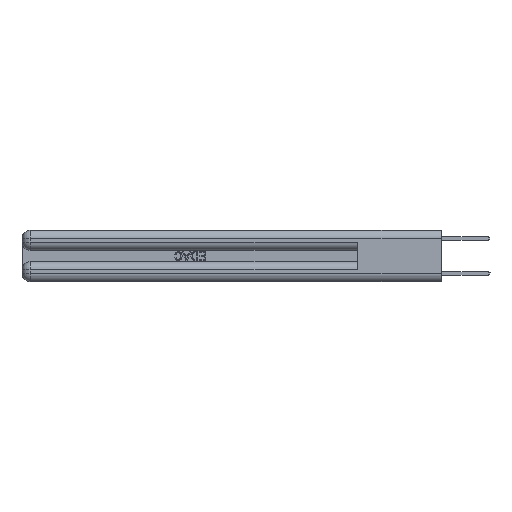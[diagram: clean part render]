
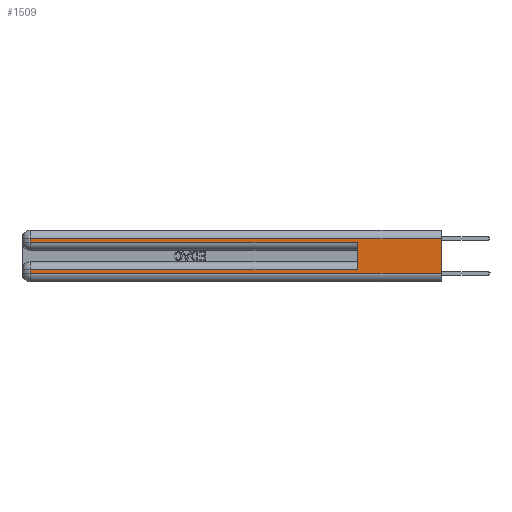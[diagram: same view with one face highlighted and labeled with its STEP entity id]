
A CAD part, left-side view. The second image highlights one B-rep face of the part: STEP entity #1509.
In plain terms, the highlighted planar face has unit normal (-1, 0, 0).
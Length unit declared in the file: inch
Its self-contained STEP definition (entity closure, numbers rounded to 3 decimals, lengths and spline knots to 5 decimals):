
#1509 = ADVANCED_FACE ( 'NONE', ( #26019 ), #21164, .F. ) ;
#1555 = VECTOR ( 'NONE', #27478, 39.37008 ) ;
#2676 = ORIENTED_EDGE ( 'NONE', *, *, #32297, .T. ) ;
#3340 = LINE ( 'NONE', #23990, #4583 ) ;
#3358 = VERTEX_POINT ( 'NONE', #25295 ) ;
#4510 = VECTOR ( 'NONE', #8321, 39.37008 ) ;
#4583 = VECTOR ( 'NONE', #26421, 39.37008 ) ;
#4674 = LINE ( 'NONE', #17213, #26048 ) ;
#5119 = VERTEX_POINT ( 'NONE', #22044 ) ;
#5182 = CARTESIAN_POINT ( 'NONE',  ( 0., 0., 0.31 ) ) ;
#6257 = DIRECTION ( 'NONE',  ( 0., 0., 1. ) ) ;
#6576 = ORIENTED_EDGE ( 'NONE', *, *, #20934, .T. ) ;
#8011 = AXIS2_PLACEMENT_3D ( 'NONE', #23850, #18541, #18206 ) ;
#8321 = DIRECTION ( 'NONE',  ( 0., 1., 0. ) ) ;
#9750 = CARTESIAN_POINT ( 'NONE',  ( 0., 2.94, 0.285 ) ) ;
#9998 = CARTESIAN_POINT ( 'NONE',  ( 0., 2.94, 0.06 ) ) ;
#10073 = LINE ( 'NONE', #34073, #13478 ) ;
#10141 = ORIENTED_EDGE ( 'NONE', *, *, #14459, .T. ) ;
#10171 = VERTEX_POINT ( 'NONE', #15647 ) ;
#10617 = VERTEX_POINT ( 'NONE', #9750 ) ;
#11072 = CARTESIAN_POINT ( 'NONE',  ( 0., 0., 0.285 ) ) ;
#11188 = DIRECTION ( 'NONE',  ( 0., -1., 0. ) ) ;
#11215 = ORIENTED_EDGE ( 'NONE', *, *, #25779, .T. ) ;
#11703 = CARTESIAN_POINT ( 'NONE',  ( 0., 0.6, 0.285 ) ) ;
#12539 = CARTESIAN_POINT ( 'NONE',  ( 0., 0.6, 0.085 ) ) ;
#13371 = ORIENTED_EDGE ( 'NONE', *, *, #18520, .F. ) ;
#13478 = VECTOR ( 'NONE', #25887, 39.37008 ) ;
#13658 = ORIENTED_EDGE ( 'NONE', *, *, #30019, .F. ) ;
#13848 = VECTOR ( 'NONE', #18808, 39.37008 ) ;
#13983 = VECTOR ( 'NONE', #29239, 39.37008 ) ;
#14459 = EDGE_CURVE ( 'NONE', #27688, #10171, #24209, .T. ) ;
#15647 = CARTESIAN_POINT ( 'NONE',  ( 0., 2.94, 0.085 ) ) ;
#15725 = EDGE_LOOP ( 'NONE', ( #13658, #6576, #2676, #28326, #13371, #10141, #11215, #18816 ) ) ;
#16240 = CARTESIAN_POINT ( 'NONE',  ( 0., 0., 0.085 ) ) ;
#16545 = LINE ( 'NONE', #18917, #13983 ) ;
#17213 = CARTESIAN_POINT ( 'NONE',  ( 0., 0.6, 0.145 ) ) ;
#18206 = DIRECTION ( 'NONE',  ( 0., 0., -1. ) ) ;
#18520 = EDGE_CURVE ( 'NONE', #27688, #21229, #4674, .T. ) ;
#18541 = DIRECTION ( 'NONE',  ( 1., 0., 0. ) ) ;
#18808 = DIRECTION ( 'NONE',  ( 0., 0., -1. ) ) ;
#18816 = ORIENTED_EDGE ( 'NONE', *, *, #27837, .T. ) ;
#18917 = CARTESIAN_POINT ( 'NONE',  ( 0., 0., 0.37 ) ) ;
#20900 = LINE ( 'NONE', #30512, #1555 ) ;
#20934 = EDGE_CURVE ( 'NONE', #26578, #3358, #3340, .T. ) ;
#21164 = PLANE ( 'NONE',  #8011 ) ;
#21229 = VERTEX_POINT ( 'NONE', #11703 ) ;
#22044 = CARTESIAN_POINT ( 'NONE',  ( 0., 0., 0.06 ) ) ;
#22834 = LINE ( 'NONE', #11072, #26942 ) ;
#23850 = CARTESIAN_POINT ( 'NONE',  ( 0., 0., 0.37 ) ) ;
#23990 = CARTESIAN_POINT ( 'NONE',  ( 0., 0., 0.31 ) ) ;
#24209 = LINE ( 'NONE', #16240, #4510 ) ;
#25295 = CARTESIAN_POINT ( 'NONE',  ( 0., 2.94, 0.31 ) ) ;
#25779 = EDGE_CURVE ( 'NONE', #10171, #33607, #10073, .T. ) ;
#25887 = DIRECTION ( 'NONE',  ( 0., 0., -1. ) ) ;
#26019 = FACE_OUTER_BOUND ( 'NONE', #15725, .T. ) ;
#26048 = VECTOR ( 'NONE', #6257, 39.37008 ) ;
#26421 = DIRECTION ( 'NONE',  ( 0., 1., 0. ) ) ;
#26578 = VERTEX_POINT ( 'NONE', #5182 ) ;
#26768 = CARTESIAN_POINT ( 'NONE',  ( 0., 2.94, 0.37 ) ) ;
#26942 = VECTOR ( 'NONE', #11188, 39.37008 ) ;
#27478 = DIRECTION ( 'NONE',  ( 0., -1., 0. ) ) ;
#27688 = VERTEX_POINT ( 'NONE', #12539 ) ;
#27837 = EDGE_CURVE ( 'NONE', #33607, #5119, #20900, .T. ) ;
#28326 = ORIENTED_EDGE ( 'NONE', *, *, #30790, .T. ) ;
#29239 = DIRECTION ( 'NONE',  ( 0., 0., -1. ) ) ;
#30019 = EDGE_CURVE ( 'NONE', #26578, #5119, #16545, .T. ) ;
#30512 = CARTESIAN_POINT ( 'NONE',  ( 0., 0., 0.06 ) ) ;
#30790 = EDGE_CURVE ( 'NONE', #10617, #21229, #22834, .T. ) ;
#32297 = EDGE_CURVE ( 'NONE', #3358, #10617, #33961, .T. ) ;
#33607 = VERTEX_POINT ( 'NONE', #9998 ) ;
#33961 = LINE ( 'NONE', #26768, #13848 ) ;
#34073 = CARTESIAN_POINT ( 'NONE',  ( 0., 2.94, 0.37 ) ) ;
